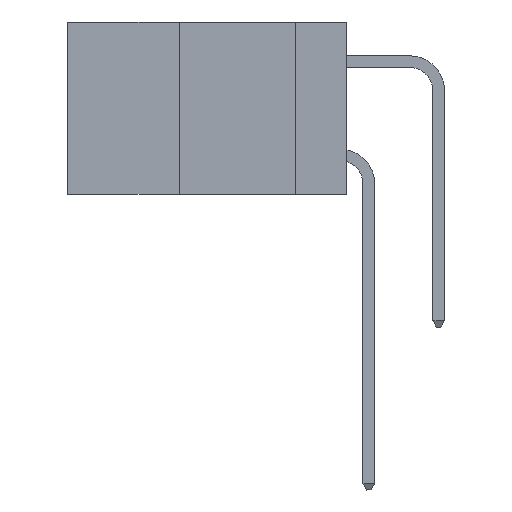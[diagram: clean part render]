
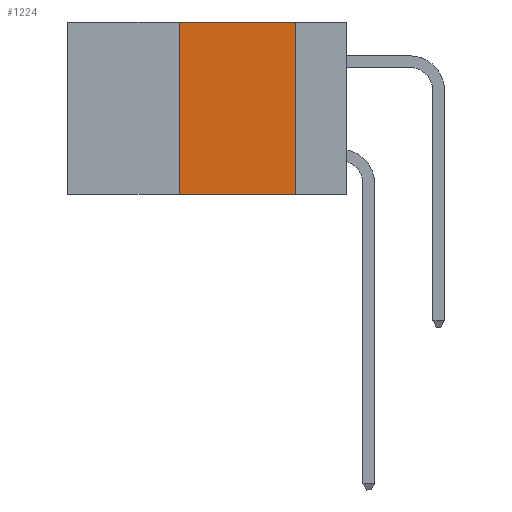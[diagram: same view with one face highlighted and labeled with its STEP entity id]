
A CAD part, left-side view. The second image highlights one B-rep face of the part: STEP entity #1224.
In plain terms, the highlighted planar face has unit normal (-1, 0, 0).
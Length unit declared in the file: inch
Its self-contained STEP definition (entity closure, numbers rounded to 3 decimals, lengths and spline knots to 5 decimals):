
#1146 = FACE_OUTER_BOUND ( 'NONE', #5886, .T. ) ;
#1224 = ADVANCED_FACE ( 'NONE', ( #1146 ), #10246, .F. ) ;
#5344 = VERTEX_POINT ( 'NONE', #10817 ) ;
#5733 = AXIS2_PLACEMENT_3D ( 'NONE', #10574, #31713, #31376 ) ;
#5880 = CARTESIAN_POINT ( 'NONE',  ( 0., 0.6, 0. ) ) ;
#5886 = EDGE_LOOP ( 'NONE', ( #17261, #23905, #33767, #23576 ) ) ;
#5995 = LINE ( 'NONE', #14977, #26128 ) ;
#6350 = LINE ( 'NONE', #5880, #19483 ) ;
#6903 = VERTEX_POINT ( 'NONE', #13314 ) ;
#8755 = DIRECTION ( 'NONE',  ( 0., -1., 0. ) ) ;
#10246 = PLANE ( 'NONE',  #5733 ) ;
#10574 = CARTESIAN_POINT ( 'NONE',  ( 0., 0.6, 0. ) ) ;
#10817 = CARTESIAN_POINT ( 'NONE',  ( 0., 0.11, 0. ) ) ;
#13314 = CARTESIAN_POINT ( 'NONE',  ( 0., 0.36, -0.37 ) ) ;
#13407 = EDGE_CURVE ( 'NONE', #6903, #22907, #16263, .T. ) ;
#13501 = EDGE_CURVE ( 'NONE', #6903, #29719, #5995, .T. ) ;
#13944 = CARTESIAN_POINT ( 'NONE',  ( 0., 0.6, -0.37 ) ) ;
#14977 = CARTESIAN_POINT ( 'NONE',  ( 0., 0.36, 0. ) ) ;
#15202 = DIRECTION ( 'NONE',  ( 0., 0., 1. ) ) ;
#16263 = LINE ( 'NONE', #13944, #20371 ) ;
#17261 = ORIENTED_EDGE ( 'NONE', *, *, #23222, .F. ) ;
#19483 = VECTOR ( 'NONE', #8755, 39.37008 ) ;
#20371 = VECTOR ( 'NONE', #33381, 39.37008 ) ;
#20457 = CARTESIAN_POINT ( 'NONE',  ( 0., 0.11, -0.37 ) ) ;
#22106 = EDGE_CURVE ( 'NONE', #29719, #5344, #6350, .T. ) ;
#22907 = VERTEX_POINT ( 'NONE', #20457 ) ;
#23222 = EDGE_CURVE ( 'NONE', #5344, #22907, #25147, .T. ) ;
#23576 = ORIENTED_EDGE ( 'NONE', *, *, #13407, .T. ) ;
#23905 = ORIENTED_EDGE ( 'NONE', *, *, #22106, .F. ) ;
#25147 = LINE ( 'NONE', #32778, #31421 ) ;
#26128 = VECTOR ( 'NONE', #15202, 39.37008 ) ;
#29719 = VERTEX_POINT ( 'NONE', #32195 ) ;
#30439 = DIRECTION ( 'NONE',  ( 0., 0., -1. ) ) ;
#31376 = DIRECTION ( 'NONE',  ( 0., 0., -1. ) ) ;
#31421 = VECTOR ( 'NONE', #30439, 39.37008 ) ;
#31713 = DIRECTION ( 'NONE',  ( 1., 0., 0. ) ) ;
#32195 = CARTESIAN_POINT ( 'NONE',  ( 0., 0.36, 0. ) ) ;
#32778 = CARTESIAN_POINT ( 'NONE',  ( 0., 0.11, 0. ) ) ;
#33381 = DIRECTION ( 'NONE',  ( 0., -1., 0. ) ) ;
#33767 = ORIENTED_EDGE ( 'NONE', *, *, #13501, .F. ) ;
